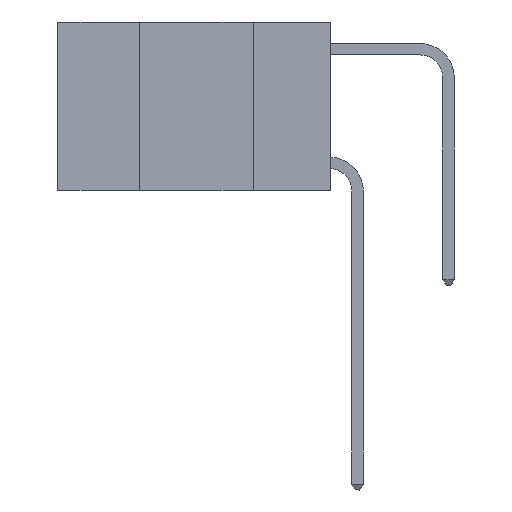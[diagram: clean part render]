
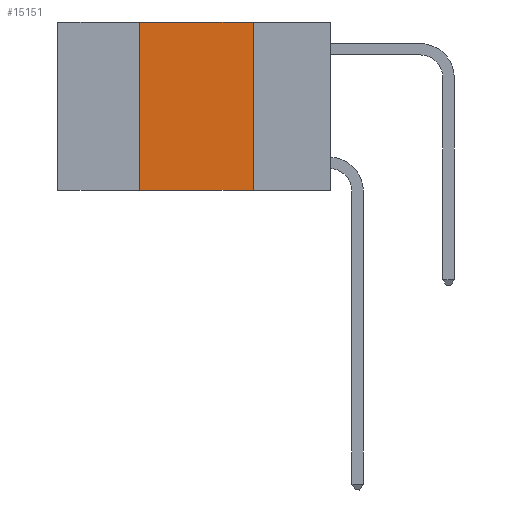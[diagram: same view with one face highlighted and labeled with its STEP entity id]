
A CAD part, left-side view. The second image highlights one B-rep face of the part: STEP entity #15151.
In plain terms, the highlighted planar face has unit normal (-1, 0, 0).
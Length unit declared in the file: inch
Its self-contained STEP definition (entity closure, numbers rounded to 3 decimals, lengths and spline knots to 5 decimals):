
#262 = CARTESIAN_POINT ( 'NONE',  ( 0., 0.42, 0. ) ) ;
#2646 = CARTESIAN_POINT ( 'NONE',  ( 0., 0.17, -0.37 ) ) ;
#3354 = VERTEX_POINT ( 'NONE', #16851 ) ;
#3641 = VERTEX_POINT ( 'NONE', #2646 ) ;
#3847 = VECTOR ( 'NONE', #6423, 39.37008 ) ;
#4064 = LINE ( 'NONE', #16773, #17987 ) ;
#4256 = AXIS2_PLACEMENT_3D ( 'NONE', #8516, #18854, #10032 ) ;
#4702 = ORIENTED_EDGE ( 'NONE', *, *, #5547, .F. ) ;
#4924 = CARTESIAN_POINT ( 'NONE',  ( 0., 0.42, 0. ) ) ;
#5231 = EDGE_CURVE ( 'NONE', #9863, #9879, #7797, .T. ) ;
#5547 = EDGE_CURVE ( 'NONE', #9879, #3354, #4064, .T. ) ;
#6423 = DIRECTION ( 'NONE',  ( 0., 0., 1. ) ) ;
#6499 = DIRECTION ( 'NONE',  ( 0., -1., 0. ) ) ;
#7797 = LINE ( 'NONE', #4924, #3847 ) ;
#8057 = LINE ( 'NONE', #9870, #11560 ) ;
#8516 = CARTESIAN_POINT ( 'NONE',  ( 0., 0.6, 0. ) ) ;
#9131 = CARTESIAN_POINT ( 'NONE',  ( 0., 0.42, -0.37 ) ) ;
#9494 = EDGE_CURVE ( 'NONE', #3354, #3641, #8057, .T. ) ;
#9751 = EDGE_LOOP ( 'NONE', ( #14733, #4702, #16775, #18614 ) ) ;
#9863 = VERTEX_POINT ( 'NONE', #9131 ) ;
#9870 = CARTESIAN_POINT ( 'NONE',  ( 0., 0.17, 0. ) ) ;
#9879 = VERTEX_POINT ( 'NONE', #262 ) ;
#9966 = PLANE ( 'NONE',  #4256 ) ;
#10032 = DIRECTION ( 'NONE',  ( 0., 0., -1. ) ) ;
#10717 = FACE_OUTER_BOUND ( 'NONE', #9751, .T. ) ;
#11560 = VECTOR ( 'NONE', #18680, 39.37008 ) ;
#11788 = VECTOR ( 'NONE', #6499, 39.37008 ) ;
#14733 = ORIENTED_EDGE ( 'NONE', *, *, #9494, .F. ) ;
#15151 = ADVANCED_FACE ( 'NONE', ( #10717 ), #9966, .F. ) ;
#15300 = DIRECTION ( 'NONE',  ( 0., -1., 0. ) ) ;
#15708 = LINE ( 'NONE', #16160, #11788 ) ;
#16160 = CARTESIAN_POINT ( 'NONE',  ( 0., 0.6, -0.37 ) ) ;
#16773 = CARTESIAN_POINT ( 'NONE',  ( 0., 0.6, 0. ) ) ;
#16775 = ORIENTED_EDGE ( 'NONE', *, *, #5231, .F. ) ;
#16851 = CARTESIAN_POINT ( 'NONE',  ( 0., 0.17, 0. ) ) ;
#17215 = EDGE_CURVE ( 'NONE', #9863, #3641, #15708, .T. ) ;
#17987 = VECTOR ( 'NONE', #15300, 39.37008 ) ;
#18614 = ORIENTED_EDGE ( 'NONE', *, *, #17215, .T. ) ;
#18680 = DIRECTION ( 'NONE',  ( 0., 0., -1. ) ) ;
#18854 = DIRECTION ( 'NONE',  ( 1., 0., 0. ) ) ;
